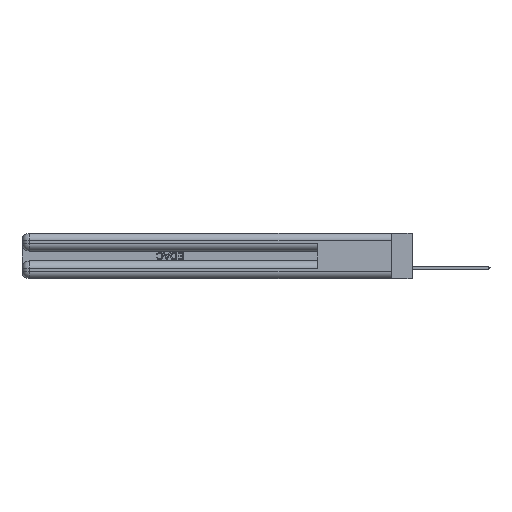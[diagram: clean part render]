
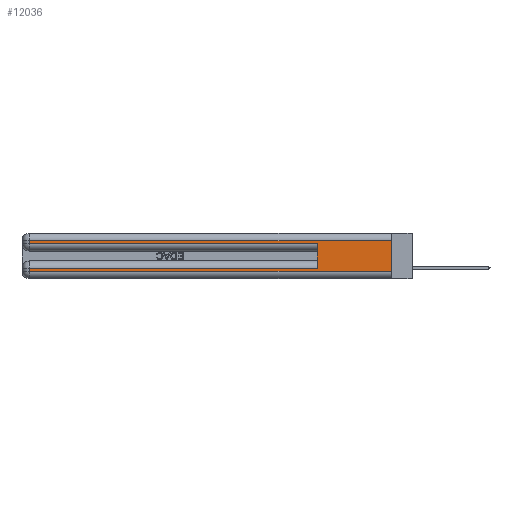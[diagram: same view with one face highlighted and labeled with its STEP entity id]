
A CAD part, left-side view. The second image highlights one B-rep face of the part: STEP entity #12036.
In plain terms, the highlighted planar face has unit normal (-1, 0, 0).
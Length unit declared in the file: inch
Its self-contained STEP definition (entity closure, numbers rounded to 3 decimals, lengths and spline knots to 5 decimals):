
#3 = VECTOR ( 'NONE', #51401, 39.37008 ) ;
#174 = VERTEX_POINT ( 'NONE', #1628 ) ;
#570 = ORIENTED_EDGE ( 'NONE', *, *, #19780, .T. ) ;
#655 = CARTESIAN_POINT ( 'NONE',  ( 0., 0., 0.285 ) ) ;
#998 = DIRECTION ( 'NONE',  ( 0., -1., 0. ) ) ;
#1472 = CARTESIAN_POINT ( 'NONE',  ( 0., 0., 0.37 ) ) ;
#1628 = CARTESIAN_POINT ( 'NONE',  ( 0., 0.6, 0.285 ) ) ;
#2972 = CARTESIAN_POINT ( 'NONE',  ( 0., 2.94, 0.085 ) ) ;
#4805 = EDGE_CURVE ( 'NONE', #7160, #39414, #23192, .T. ) ;
#5758 = EDGE_CURVE ( 'NONE', #25596, #32298, #47399, .T. ) ;
#6194 = DIRECTION ( 'NONE',  ( 0., 0., -1. ) ) ;
#7160 = VERTEX_POINT ( 'NONE', #46926 ) ;
#7818 = EDGE_LOOP ( 'NONE', ( #34186, #32234, #37905, #39733, #21825, #36785, #45310, #570 ) ) ;
#10429 = VERTEX_POINT ( 'NONE', #39559 ) ;
#12036 = ADVANCED_FACE ( 'NONE', ( #12405 ), #37573, .F. ) ;
#12405 = FACE_OUTER_BOUND ( 'NONE', #7818, .T. ) ;
#15013 = LINE ( 'NONE', #655, #21232 ) ;
#16126 = CARTESIAN_POINT ( 'NONE',  ( 0., 2.94, 0.31 ) ) ;
#16925 = EDGE_CURVE ( 'NONE', #10429, #174, #15013, .T. ) ;
#18970 = CARTESIAN_POINT ( 'NONE',  ( 0., 0., 0.37 ) ) ;
#19780 = EDGE_CURVE ( 'NONE', #37386, #40622, #44343, .T. ) ;
#21232 = VECTOR ( 'NONE', #998, 39.37008 ) ;
#21460 = CARTESIAN_POINT ( 'NONE',  ( 0., 0., 0.31 ) ) ;
#21825 = ORIENTED_EDGE ( 'NONE', *, *, #29771, .F. ) ;
#21997 = DIRECTION ( 'NONE',  ( 0., 1., 0. ) ) ;
#22870 = VECTOR ( 'NONE', #21997, 39.37008 ) ;
#23192 = LINE ( 'NONE', #50402, #26336 ) ;
#23808 = CARTESIAN_POINT ( 'NONE',  ( 0., 2.94, 0.37 ) ) ;
#24891 = LINE ( 'NONE', #18970, #25405 ) ;
#25405 = VECTOR ( 'NONE', #32341, 39.37008 ) ;
#25501 = CARTESIAN_POINT ( 'NONE',  ( 0., 2.94, 0.06 ) ) ;
#25530 = DIRECTION ( 'NONE',  ( 1., 0., 0. ) ) ;
#25596 = VERTEX_POINT ( 'NONE', #28214 ) ;
#26336 = VECTOR ( 'NONE', #37934, 39.37008 ) ;
#28164 = LINE ( 'NONE', #23808, #47648 ) ;
#28214 = CARTESIAN_POINT ( 'NONE',  ( 0., 0., 0.31 ) ) ;
#28683 = EDGE_CURVE ( 'NONE', #32298, #10429, #28164, .T. ) ;
#29771 = EDGE_CURVE ( 'NONE', #7160, #174, #30525, .T. ) ;
#29878 = CARTESIAN_POINT ( 'NONE',  ( 0., 2.94, 0.37 ) ) ;
#30053 = DIRECTION ( 'NONE',  ( 0., -1., 0. ) ) ;
#30525 = LINE ( 'NONE', #38778, #3 ) ;
#32234 = ORIENTED_EDGE ( 'NONE', *, *, #5758, .T. ) ;
#32298 = VERTEX_POINT ( 'NONE', #16126 ) ;
#32341 = DIRECTION ( 'NONE',  ( 0., 0., -1. ) ) ;
#32435 = AXIS2_PLACEMENT_3D ( 'NONE', #1472, #25530, #6194 ) ;
#33915 = DIRECTION ( 'NONE',  ( 0., 0., -1. ) ) ;
#34186 = ORIENTED_EDGE ( 'NONE', *, *, #49383, .F. ) ;
#34980 = VECTOR ( 'NONE', #30053, 39.37008 ) ;
#35144 = CARTESIAN_POINT ( 'NONE',  ( 0., 0., 0.06 ) ) ;
#36785 = ORIENTED_EDGE ( 'NONE', *, *, #4805, .T. ) ;
#37386 = VERTEX_POINT ( 'NONE', #25501 ) ;
#37573 = PLANE ( 'NONE',  #32435 ) ;
#37723 = CARTESIAN_POINT ( 'NONE',  ( 0., 0., 0.06 ) ) ;
#37905 = ORIENTED_EDGE ( 'NONE', *, *, #28683, .T. ) ;
#37934 = DIRECTION ( 'NONE',  ( 0., 1., 0. ) ) ;
#38778 = CARTESIAN_POINT ( 'NONE',  ( 0., 0.6, 0.145 ) ) ;
#39414 = VERTEX_POINT ( 'NONE', #2972 ) ;
#39559 = CARTESIAN_POINT ( 'NONE',  ( 0., 2.94, 0.285 ) ) ;
#39733 = ORIENTED_EDGE ( 'NONE', *, *, #16925, .T. ) ;
#40622 = VERTEX_POINT ( 'NONE', #35144 ) ;
#42665 = VECTOR ( 'NONE', #33915, 39.37008 ) ;
#44343 = LINE ( 'NONE', #37723, #34980 ) ;
#44593 = DIRECTION ( 'NONE',  ( 0., 0., -1. ) ) ;
#45103 = EDGE_CURVE ( 'NONE', #39414, #37386, #47046, .T. ) ;
#45310 = ORIENTED_EDGE ( 'NONE', *, *, #45103, .T. ) ;
#46926 = CARTESIAN_POINT ( 'NONE',  ( 0., 0.6, 0.085 ) ) ;
#47046 = LINE ( 'NONE', #29878, #42665 ) ;
#47399 = LINE ( 'NONE', #21460, #22870 ) ;
#47648 = VECTOR ( 'NONE', #44593, 39.37008 ) ;
#49383 = EDGE_CURVE ( 'NONE', #25596, #40622, #24891, .T. ) ;
#50402 = CARTESIAN_POINT ( 'NONE',  ( 0., 0., 0.085 ) ) ;
#51401 = DIRECTION ( 'NONE',  ( 0., 0., 1. ) ) ;
